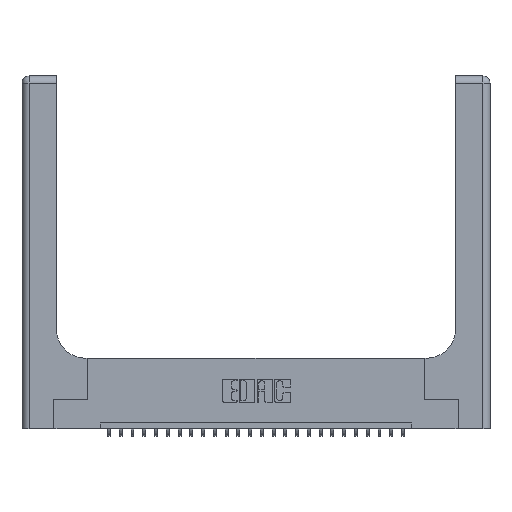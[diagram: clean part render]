
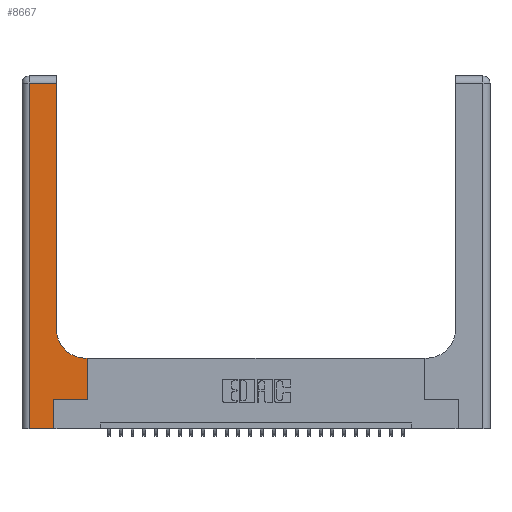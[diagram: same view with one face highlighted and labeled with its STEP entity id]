
A CAD part, top view. The second image highlights one B-rep face of the part: STEP entity #8667.
In plain terms, the highlighted planar face has unit normal (0, 0, 1).
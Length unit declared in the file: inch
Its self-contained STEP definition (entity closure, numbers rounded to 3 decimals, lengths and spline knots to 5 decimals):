
#1028 = VECTOR ( 'NONE', #2557, 39.37008 ) ;
#1458 = FACE_OUTER_BOUND ( 'NONE', #21293, .T. ) ;
#1531 = CARTESIAN_POINT ( 'NONE',  ( 0.5585, 0.25, 0.37 ) ) ;
#2557 = DIRECTION ( 'NONE',  ( 1., 0., 0. ) ) ;
#2895 = CARTESIAN_POINT ( 'NONE',  ( 0., 3., 0.37 ) ) ;
#3755 = LINE ( 'NONE', #12003, #24925 ) ;
#4042 = AXIS2_PLACEMENT_3D ( 'NONE', #2895, #23652, #23305 ) ;
#4079 = VERTEX_POINT ( 'NONE', #22409 ) ;
#4942 = ORIENTED_EDGE ( 'NONE', *, *, #26303, .T. ) ;
#5149 = VERTEX_POINT ( 'NONE', #25935 ) ;
#5816 = LINE ( 'NONE', #18075, #8732 ) ;
#6004 = DIRECTION ( 'NONE',  ( 1., 0., 0. ) ) ;
#6255 = EDGE_CURVE ( 'NONE', #11149, #23648, #23387, .T. ) ;
#6929 = DIRECTION ( 'NONE',  ( -1., 0., 0. ) ) ;
#7571 = EDGE_CURVE ( 'NONE', #23648, #16432, #7726, .T. ) ;
#7617 = LINE ( 'NONE', #13422, #22583 ) ;
#7726 = LINE ( 'NONE', #14307, #25603 ) ;
#8667 = ADVANCED_FACE ( 'NONE', ( #1458 ), #17429, .F. ) ;
#8732 = VECTOR ( 'NONE', #16073, 39.37008 ) ;
#9002 = CARTESIAN_POINT ( 'NONE',  ( 0.269, 0.25, 0.37 ) ) ;
#10364 = CARTESIAN_POINT ( 'NONE',  ( 0.06, 0., 0.37 ) ) ;
#10373 = CARTESIAN_POINT ( 'NONE',  ( 0., 0., 0.37 ) ) ;
#10454 = VECTOR ( 'NONE', #22708, 39.37008 ) ;
#10469 = EDGE_CURVE ( 'NONE', #18965, #11149, #20299, .T. ) ;
#11149 = VERTEX_POINT ( 'NONE', #17810 ) ;
#12003 = CARTESIAN_POINT ( 'NONE',  ( 0.2915, 0.6, 0.37 ) ) ;
#12532 = EDGE_CURVE ( 'NONE', #24302, #18965, #5816, .T. ) ;
#13190 = VERTEX_POINT ( 'NONE', #21751 ) ;
#13422 = CARTESIAN_POINT ( 'NONE',  ( 0., 2.94, 0.37 ) ) ;
#13911 = ORIENTED_EDGE ( 'NONE', *, *, #16486, .T. ) ;
#13953 = VECTOR ( 'NONE', #23845, 39.37008 ) ;
#14131 = DIRECTION ( 'NONE',  ( 0., 0., -1. ) ) ;
#14307 = CARTESIAN_POINT ( 'NONE',  ( 0.269, 0.25, 0.37 ) ) ;
#14655 = ORIENTED_EDGE ( 'NONE', *, *, #18484, .T. ) ;
#14933 = ORIENTED_EDGE ( 'NONE', *, *, #17115, .T. ) ;
#16073 = DIRECTION ( 'NONE',  ( 0., -1., 0. ) ) ;
#16254 = DIRECTION ( 'NONE',  ( -1., 0., 0. ) ) ;
#16432 = VERTEX_POINT ( 'NONE', #1531 ) ;
#16486 = EDGE_CURVE ( 'NONE', #13190, #4079, #20950, .T. ) ;
#17115 = EDGE_CURVE ( 'NONE', #16432, #20914, #17356, .T. ) ;
#17356 = LINE ( 'NONE', #18489, #10454 ) ;
#17429 = PLANE ( 'NONE',  #4042 ) ;
#17443 = CARTESIAN_POINT ( 'NONE',  ( 0.269, 0., 0.37 ) ) ;
#17576 = ORIENTED_EDGE ( 'NONE', *, *, #12532, .T. ) ;
#17614 = ORIENTED_EDGE ( 'NONE', *, *, #7571, .T. ) ;
#17810 = CARTESIAN_POINT ( 'NONE',  ( 0.269, 0., 0.37 ) ) ;
#18075 = CARTESIAN_POINT ( 'NONE',  ( 0.06, 3., 0.37 ) ) ;
#18484 = EDGE_CURVE ( 'NONE', #5149, #24302, #7617, .T. ) ;
#18489 = CARTESIAN_POINT ( 'NONE',  ( 0.5585, 0.25, 0.37 ) ) ;
#18965 = VERTEX_POINT ( 'NONE', #10364 ) ;
#20299 = LINE ( 'NONE', #10373, #1028 ) ;
#20597 = CARTESIAN_POINT ( 'NONE',  ( 0.5415, 0.85, 0.37 ) ) ;
#20688 = ORIENTED_EDGE ( 'NONE', *, *, #10469, .T. ) ;
#20914 = VERTEX_POINT ( 'NONE', #23877 ) ;
#20950 = CIRCLE ( 'NONE', #24657, 0.25 ) ;
#20951 = DIRECTION ( 'NONE',  ( 0., 1., 0. ) ) ;
#21216 = ORIENTED_EDGE ( 'NONE', *, *, #23874, .T. ) ;
#21293 = EDGE_LOOP ( 'NONE', ( #4942, #14655, #17576, #20688, #24541, #17614, #14933, #21216, #13911 ) ) ;
#21751 = CARTESIAN_POINT ( 'NONE',  ( 0.5415, 0.6, 0.37 ) ) ;
#21835 = CARTESIAN_POINT ( 'NONE',  ( 0.06, 2.94, 0.37 ) ) ;
#22409 = CARTESIAN_POINT ( 'NONE',  ( 0.2915, 0.85, 0.37 ) ) ;
#22449 = VECTOR ( 'NONE', #20951, 39.37008 ) ;
#22583 = VECTOR ( 'NONE', #6929, 39.37008 ) ;
#22708 = DIRECTION ( 'NONE',  ( 0., 1., 0. ) ) ;
#22831 = CARTESIAN_POINT ( 'NONE',  ( 0.2915, 3., 0.37 ) ) ;
#22913 = DIRECTION ( 'NONE',  ( 1., 0., 0. ) ) ;
#23305 = DIRECTION ( 'NONE',  ( -1., 0., 0. ) ) ;
#23387 = LINE ( 'NONE', #17443, #13953 ) ;
#23648 = VERTEX_POINT ( 'NONE', #9002 ) ;
#23652 = DIRECTION ( 'NONE',  ( 0., 0., -1. ) ) ;
#23845 = DIRECTION ( 'NONE',  ( 0., 1., 0. ) ) ;
#23874 = EDGE_CURVE ( 'NONE', #20914, #13190, #3755, .T. ) ;
#23877 = CARTESIAN_POINT ( 'NONE',  ( 0.5585, 0.6, 0.37 ) ) ;
#24302 = VERTEX_POINT ( 'NONE', #21835 ) ;
#24392 = LINE ( 'NONE', #22831, #22449 ) ;
#24541 = ORIENTED_EDGE ( 'NONE', *, *, #6255, .T. ) ;
#24657 = AXIS2_PLACEMENT_3D ( 'NONE', #20597, #14131, #6004 ) ;
#24925 = VECTOR ( 'NONE', #16254, 39.37008 ) ;
#25603 = VECTOR ( 'NONE', #22913, 39.37008 ) ;
#25935 = CARTESIAN_POINT ( 'NONE',  ( 0.2915, 2.94, 0.37 ) ) ;
#26303 = EDGE_CURVE ( 'NONE', #4079, #5149, #24392, .T. ) ;
